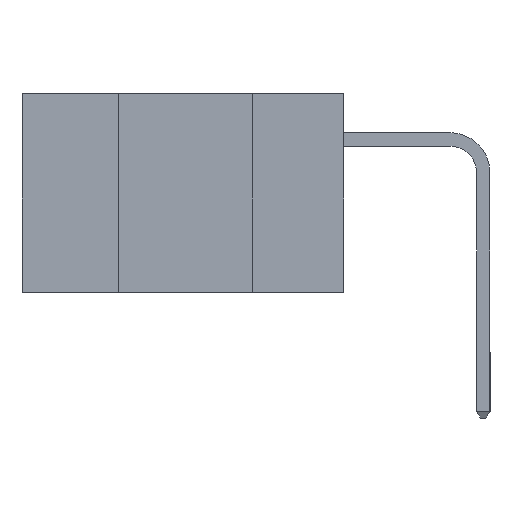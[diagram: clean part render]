
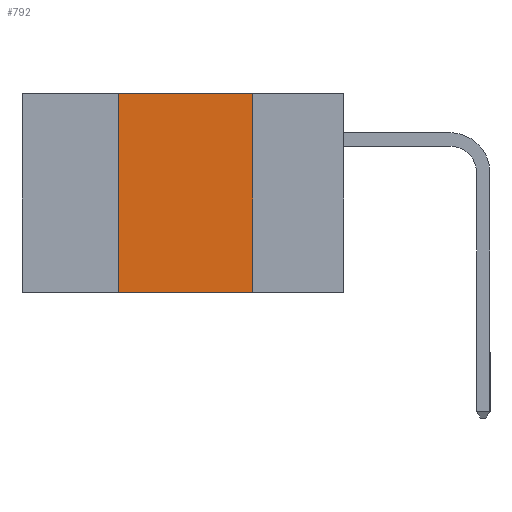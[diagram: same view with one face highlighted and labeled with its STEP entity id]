
A CAD part, left-side view. The second image highlights one B-rep face of the part: STEP entity #792.
In plain terms, the highlighted planar face has unit normal (-1, 0, 0).
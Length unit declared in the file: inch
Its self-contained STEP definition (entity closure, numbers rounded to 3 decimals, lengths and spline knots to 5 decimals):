
#792 = ADVANCED_FACE ( 'NONE', ( #4305 ), #9310, .F. ) ;
#1563 = DIRECTION ( 'NONE',  ( 0., 0., -1. ) ) ;
#1662 = CARTESIAN_POINT ( 'NONE',  ( 0., 0.17, 0. ) ) ;
#2178 = VERTEX_POINT ( 'NONE', #11333 ) ;
#2772 = CARTESIAN_POINT ( 'NONE',  ( 0., 0.17, 0. ) ) ;
#3096 = CARTESIAN_POINT ( 'NONE',  ( 0., 0.6, 0. ) ) ;
#3353 = DIRECTION ( 'NONE',  ( 0., -1., 0. ) ) ;
#3549 = EDGE_CURVE ( 'NONE', #11446, #11332, #8287, .T. ) ;
#3558 = VECTOR ( 'NONE', #1563, 39.37008 ) ;
#3573 = ORIENTED_EDGE ( 'NONE', *, *, #4293, .T. ) ;
#3985 = ORIENTED_EDGE ( 'NONE', *, *, #16670, .F. ) ;
#4163 = DIRECTION ( 'NONE',  ( 0., 0., -1. ) ) ;
#4293 = EDGE_CURVE ( 'NONE', #12476, #2178, #5410, .T. ) ;
#4305 = FACE_OUTER_BOUND ( 'NONE', #10856, .T. ) ;
#5410 = LINE ( 'NONE', #16375, #10214 ) ;
#5496 = DIRECTION ( 'NONE',  ( 0., -1., 0. ) ) ;
#7866 = VECTOR ( 'NONE', #5496, 39.37008 ) ;
#8287 = LINE ( 'NONE', #3096, #7866 ) ;
#9310 = PLANE ( 'NONE',  #16566 ) ;
#9762 = LINE ( 'NONE', #11076, #15998 ) ;
#10072 = DIRECTION ( 'NONE',  ( 0., 0., 1. ) ) ;
#10214 = VECTOR ( 'NONE', #3353, 39.37008 ) ;
#10387 = EDGE_CURVE ( 'NONE', #11332, #2178, #13820, .T. ) ;
#10458 = CARTESIAN_POINT ( 'NONE',  ( 0., 0.6, 0. ) ) ;
#10849 = ORIENTED_EDGE ( 'NONE', *, *, #10387, .F. ) ;
#10856 = EDGE_LOOP ( 'NONE', ( #10849, #15066, #3985, #3573 ) ) ;
#11076 = CARTESIAN_POINT ( 'NONE',  ( 0., 0.42, 0. ) ) ;
#11332 = VERTEX_POINT ( 'NONE', #1662 ) ;
#11333 = CARTESIAN_POINT ( 'NONE',  ( 0., 0.17, -0.37 ) ) ;
#11446 = VERTEX_POINT ( 'NONE', #13607 ) ;
#12476 = VERTEX_POINT ( 'NONE', #15734 ) ;
#13607 = CARTESIAN_POINT ( 'NONE',  ( 0., 0.42, 0. ) ) ;
#13820 = LINE ( 'NONE', #2772, #3558 ) ;
#15066 = ORIENTED_EDGE ( 'NONE', *, *, #3549, .F. ) ;
#15705 = DIRECTION ( 'NONE',  ( 1., 0., 0. ) ) ;
#15734 = CARTESIAN_POINT ( 'NONE',  ( 0., 0.42, -0.37 ) ) ;
#15998 = VECTOR ( 'NONE', #10072, 39.37008 ) ;
#16375 = CARTESIAN_POINT ( 'NONE',  ( 0., 0.6, -0.37 ) ) ;
#16566 = AXIS2_PLACEMENT_3D ( 'NONE', #10458, #15705, #4163 ) ;
#16670 = EDGE_CURVE ( 'NONE', #12476, #11446, #9762, .T. ) ;
